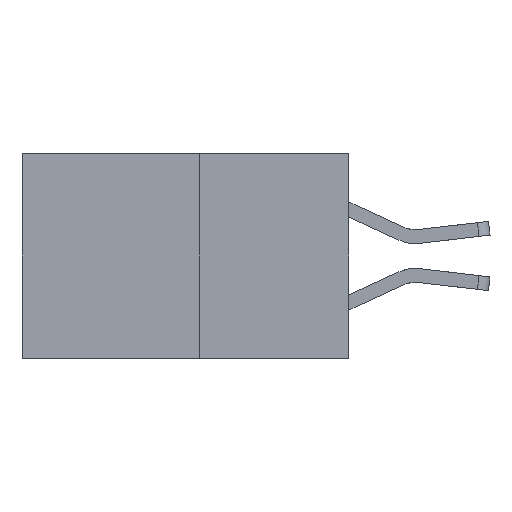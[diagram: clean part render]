
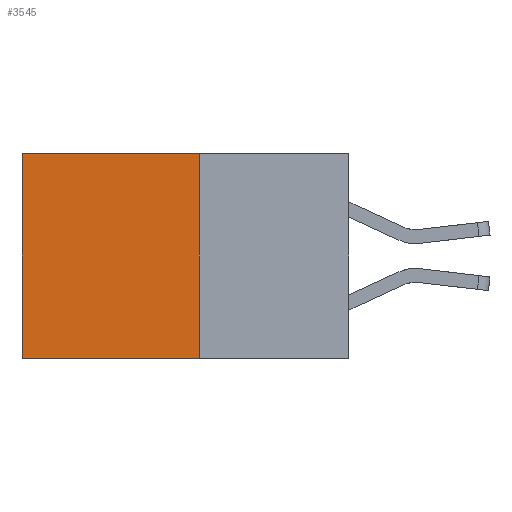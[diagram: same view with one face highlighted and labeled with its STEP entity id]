
A CAD part, left-side view. The second image highlights one B-rep face of the part: STEP entity #3545.
In plain terms, the highlighted planar face has unit normal (-1, 0, 0).
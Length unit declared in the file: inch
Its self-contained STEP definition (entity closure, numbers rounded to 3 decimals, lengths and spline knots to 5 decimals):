
#3 = ORIENTED_EDGE ( 'NONE', *, *, #9456, .T. ) ;
#101 = DIRECTION ( 'NONE',  ( 0., 0., -1. ) ) ;
#104 = DIRECTION ( 'NONE',  ( 0., 1., 0. ) ) ;
#425 = VECTOR ( 'NONE', #9243, 39.37008 ) ;
#508 = VERTEX_POINT ( 'NONE', #2863 ) ;
#797 = CARTESIAN_POINT ( 'NONE',  ( 0.277, 0.27, -0.37 ) ) ;
#1277 = EDGE_CURVE ( 'NONE', #10776, #2894, #3007, .T. ) ;
#1516 = ORIENTED_EDGE ( 'NONE', *, *, #1277, .F. ) ;
#1966 = CARTESIAN_POINT ( 'NONE',  ( 0.277, 0.27, 0. ) ) ;
#2222 = DIRECTION ( 'NONE',  ( 0., 0., -1. ) ) ;
#2819 = FACE_OUTER_BOUND ( 'NONE', #6699, .T. ) ;
#2863 = CARTESIAN_POINT ( 'NONE',  ( 0.277, 0.59, -0.37 ) ) ;
#2894 = VERTEX_POINT ( 'NONE', #10461 ) ;
#3007 = LINE ( 'NONE', #9186, #425 ) ;
#3545 = ADVANCED_FACE ( 'NONE', ( #2819 ), #4128, .F. ) ;
#3993 = CARTESIAN_POINT ( 'NONE',  ( 0.277, 0.27, 0. ) ) ;
#4128 = PLANE ( 'NONE',  #10838 ) ;
#4419 = LINE ( 'NONE', #797, #6783 ) ;
#4763 = ORIENTED_EDGE ( 'NONE', *, *, #10589, .F. ) ;
#4975 = VERTEX_POINT ( 'NONE', #11077 ) ;
#5672 = EDGE_CURVE ( 'NONE', #4975, #508, #7024, .T. ) ;
#6024 = ORIENTED_EDGE ( 'NONE', *, *, #5672, .T. ) ;
#6699 = EDGE_LOOP ( 'NONE', ( #6024, #4763, #1516, #3 ) ) ;
#6783 = VECTOR ( 'NONE', #7739, 39.37008 ) ;
#6792 = VECTOR ( 'NONE', #104, 39.37008 ) ;
#7024 = LINE ( 'NONE', #11917, #7654 ) ;
#7654 = VECTOR ( 'NONE', #101, 39.37008 ) ;
#7739 = DIRECTION ( 'NONE',  ( 0., 1., 0. ) ) ;
#7972 = CARTESIAN_POINT ( 'NONE',  ( 0.277, 0.27, -0.37 ) ) ;
#9186 = CARTESIAN_POINT ( 'NONE',  ( 0.277, 0.27, -0.37 ) ) ;
#9243 = DIRECTION ( 'NONE',  ( 0., 0., -1. ) ) ;
#9456 = EDGE_CURVE ( 'NONE', #10776, #4975, #12101, .T. ) ;
#10461 = CARTESIAN_POINT ( 'NONE',  ( 0.277, 0.27, -0.37 ) ) ;
#10589 = EDGE_CURVE ( 'NONE', #2894, #508, #4419, .T. ) ;
#10776 = VERTEX_POINT ( 'NONE', #1966 ) ;
#10838 = AXIS2_PLACEMENT_3D ( 'NONE', #7972, #12554, #2222 ) ;
#11077 = CARTESIAN_POINT ( 'NONE',  ( 0.277, 0.59, 0. ) ) ;
#11917 = CARTESIAN_POINT ( 'NONE',  ( 0.277, 0.59, -0.37 ) ) ;
#12101 = LINE ( 'NONE', #3993, #6792 ) ;
#12554 = DIRECTION ( 'NONE',  ( 1., 0., 0. ) ) ;
